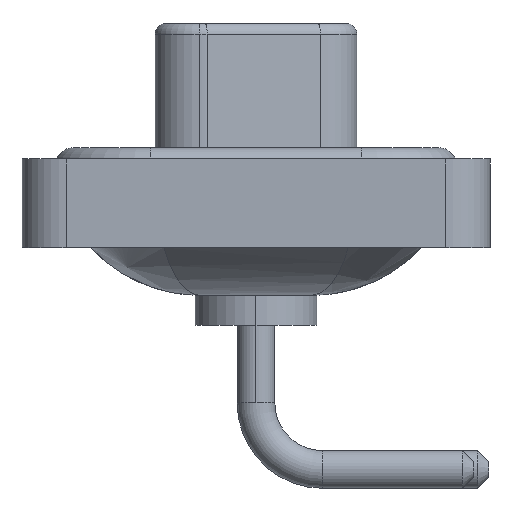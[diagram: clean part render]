
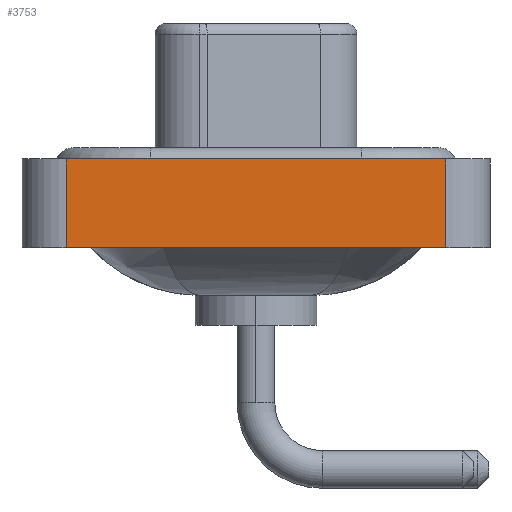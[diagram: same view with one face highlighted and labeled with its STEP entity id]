
A CAD part, left-side view. The second image highlights one B-rep face of the part: STEP entity #3753.
In plain terms, the highlighted planar face has unit normal (-1, 0, 0).
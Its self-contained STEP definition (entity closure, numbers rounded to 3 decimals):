
#834 = VERTEX_POINT ( 'NONE', #845 ) ;
#845 = CARTESIAN_POINT ( 'NONE',  ( -7.3, -8.55, -3.6 ) ) ;
#2318 = VECTOR ( 'NONE', #17224, 1000. ) ;
#3753 = ADVANCED_FACE ( 'NONE', ( #12720 ), #14358, .T. ) ;
#4905 = LINE ( 'NONE', #12286, #17012 ) ;
#6522 = VERTEX_POINT ( 'NONE', #13235 ) ;
#6750 = LINE ( 'NONE', #11268, #2318 ) ;
#7409 = EDGE_CURVE ( 'NONE', #12998, #6522, #10474, .T. ) ;
#8081 = CARTESIAN_POINT ( 'NONE',  ( -7.3, -8.55, 0.4 ) ) ;
#8480 = DIRECTION ( 'NONE',  ( 0., -1., 0. ) ) ;
#8904 = VECTOR ( 'NONE', #8480, 1000. ) ;
#10049 = ORIENTED_EDGE ( 'NONE', *, *, #7409, .F. ) ;
#10270 = CARTESIAN_POINT ( 'NONE',  ( -7.3, 8.55, -3.6 ) ) ;
#10474 = LINE ( 'NONE', #10270, #13984 ) ;
#11246 = CARTESIAN_POINT ( 'NONE',  ( -7.3, -8.55, -3.6 ) ) ;
#11268 = CARTESIAN_POINT ( 'NONE',  ( -7.3, -8.55, -3.6 ) ) ;
#11448 = DIRECTION ( 'NONE',  ( 0., 0., 1. ) ) ;
#12286 = CARTESIAN_POINT ( 'NONE',  ( -7.3, -8.55, -3.6 ) ) ;
#12720 = FACE_OUTER_BOUND ( 'NONE', #13969, .T. ) ;
#12941 = AXIS2_PLACEMENT_3D ( 'NONE', #11246, #17205, #11448 ) ;
#12998 = VERTEX_POINT ( 'NONE', #14877 ) ;
#13220 = VERTEX_POINT ( 'NONE', #8081 ) ;
#13235 = CARTESIAN_POINT ( 'NONE',  ( -7.3, 8.55, 0.4 ) ) ;
#13969 = EDGE_LOOP ( 'NONE', ( #18847, #15313, #10049, #19203 ) ) ;
#13984 = VECTOR ( 'NONE', #16241, 1000. ) ;
#14048 = EDGE_CURVE ( 'NONE', #834, #13220, #4905, .T. ) ;
#14358 = PLANE ( 'NONE',  #12941 ) ;
#14483 = EDGE_CURVE ( 'NONE', #6522, #13220, #15742, .T. ) ;
#14877 = CARTESIAN_POINT ( 'NONE',  ( -7.3, 8.55, -3.6 ) ) ;
#15313 = ORIENTED_EDGE ( 'NONE', *, *, #14483, .F. ) ;
#15742 = LINE ( 'NONE', #16038, #8904 ) ;
#16038 = CARTESIAN_POINT ( 'NONE',  ( -7.3, -8.55, 0.4 ) ) ;
#16241 = DIRECTION ( 'NONE',  ( 0., 0., 1. ) ) ;
#16863 = DIRECTION ( 'NONE',  ( 0., 0., 1. ) ) ;
#17012 = VECTOR ( 'NONE', #16863, 1000. ) ;
#17205 = DIRECTION ( 'NONE',  ( -1., 0., 0. ) ) ;
#17224 = DIRECTION ( 'NONE',  ( 0., -1., 0. ) ) ;
#18255 = EDGE_CURVE ( 'NONE', #12998, #834, #6750, .T. ) ;
#18847 = ORIENTED_EDGE ( 'NONE', *, *, #14048, .T. ) ;
#19203 = ORIENTED_EDGE ( 'NONE', *, *, #18255, .T. ) ;
